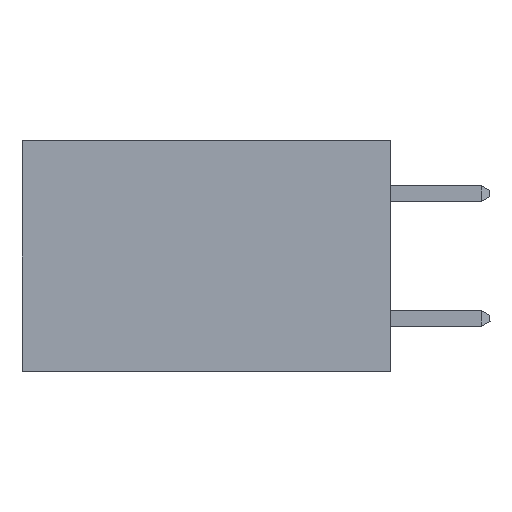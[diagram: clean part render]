
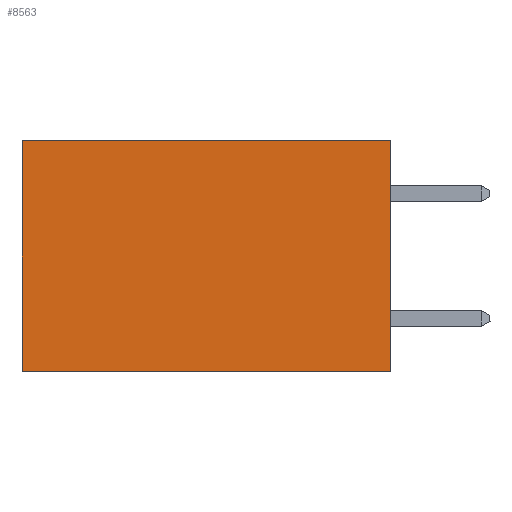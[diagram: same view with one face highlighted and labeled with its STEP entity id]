
A CAD part, left-side view. The second image highlights one B-rep face of the part: STEP entity #8563.
In plain terms, the highlighted planar face has unit normal (-1, 0, 0).
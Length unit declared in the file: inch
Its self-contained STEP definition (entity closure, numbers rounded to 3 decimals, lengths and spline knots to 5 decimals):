
#2155 = CARTESIAN_POINT ( 'NONE',  ( 0.277, 0., -0.37 ) ) ;
#2518 = DIRECTION ( 'NONE',  ( 0., 0., -1. ) ) ;
#3000 = CARTESIAN_POINT ( 'NONE',  ( 0.277, 0., -0.37 ) ) ;
#3033 = EDGE_CURVE ( 'NONE', #13506, #10284, #11555, .T. ) ;
#3213 = VECTOR ( 'NONE', #8456, 39.37008 ) ;
#3483 = ORIENTED_EDGE ( 'NONE', *, *, #3033, .T. ) ;
#3684 = LINE ( 'NONE', #3000, #7200 ) ;
#3924 = DIRECTION ( 'NONE',  ( 0., 0., -1. ) ) ;
#3963 = DIRECTION ( 'NONE',  ( 0., 1., 0. ) ) ;
#4280 = CARTESIAN_POINT ( 'NONE',  ( 0.277, 0.59, -0.37 ) ) ;
#4649 = ORIENTED_EDGE ( 'NONE', *, *, #14196, .T. ) ;
#5820 = CARTESIAN_POINT ( 'NONE',  ( 0.277, 0., 0. ) ) ;
#6276 = LINE ( 'NONE', #5820, #3213 ) ;
#6304 = FACE_OUTER_BOUND ( 'NONE', #15824, .T. ) ;
#7200 = VECTOR ( 'NONE', #12144, 39.37008 ) ;
#7658 = CARTESIAN_POINT ( 'NONE',  ( 0.277, 0., -0.37 ) ) ;
#8456 = DIRECTION ( 'NONE',  ( 0., 1., 0. ) ) ;
#8563 = ADVANCED_FACE ( 'NONE', ( #6304 ), #12879, .F. ) ;
#9309 = VECTOR ( 'NONE', #3924, 39.37008 ) ;
#10098 = CARTESIAN_POINT ( 'NONE',  ( 0.277, 0., 0. ) ) ;
#10284 = VERTEX_POINT ( 'NONE', #16062 ) ;
#10308 = DIRECTION ( 'NONE',  ( 1., 0., 0. ) ) ;
#10466 = VERTEX_POINT ( 'NONE', #2155 ) ;
#11097 = CARTESIAN_POINT ( 'NONE',  ( 0.277, 0.59, 0. ) ) ;
#11103 = AXIS2_PLACEMENT_3D ( 'NONE', #16833, #10308, #2518 ) ;
#11368 = EDGE_CURVE ( 'NONE', #10466, #10284, #11927, .T. ) ;
#11510 = VECTOR ( 'NONE', #3963, 39.37008 ) ;
#11555 = LINE ( 'NONE', #4280, #9309 ) ;
#11927 = LINE ( 'NONE', #7658, #11510 ) ;
#12025 = ORIENTED_EDGE ( 'NONE', *, *, #12253, .F. ) ;
#12144 = DIRECTION ( 'NONE',  ( 0., 0., -1. ) ) ;
#12253 = EDGE_CURVE ( 'NONE', #15720, #10466, #3684, .T. ) ;
#12750 = ORIENTED_EDGE ( 'NONE', *, *, #11368, .F. ) ;
#12879 = PLANE ( 'NONE',  #11103 ) ;
#13506 = VERTEX_POINT ( 'NONE', #11097 ) ;
#14196 = EDGE_CURVE ( 'NONE', #15720, #13506, #6276, .T. ) ;
#15720 = VERTEX_POINT ( 'NONE', #10098 ) ;
#15824 = EDGE_LOOP ( 'NONE', ( #3483, #12750, #12025, #4649 ) ) ;
#16062 = CARTESIAN_POINT ( 'NONE',  ( 0.277, 0.59, -0.37 ) ) ;
#16833 = CARTESIAN_POINT ( 'NONE',  ( 0.277, 0., -0.37 ) ) ;
